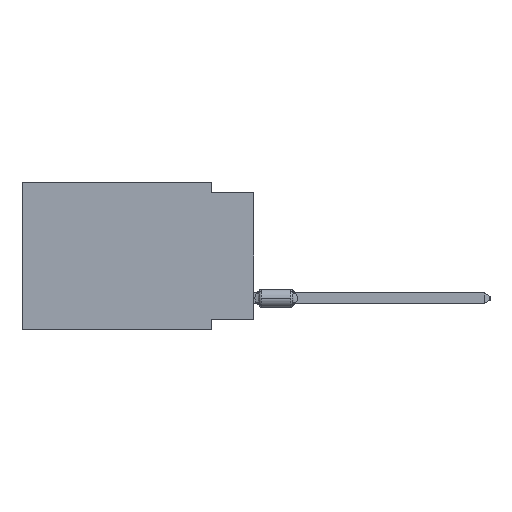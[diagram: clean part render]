
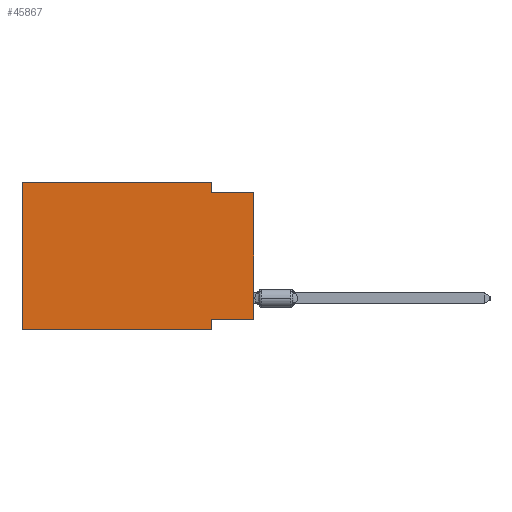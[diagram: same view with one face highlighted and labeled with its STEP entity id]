
A CAD part, left-side view. The second image highlights one B-rep face of the part: STEP entity #45867.
In plain terms, the highlighted planar face has unit normal (-1, 0, 0).
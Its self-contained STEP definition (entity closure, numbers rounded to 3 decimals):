
#582 = EDGE_CURVE ( 'NONE', #38500, #36623, #30276, .T. ) ;
#1065 = LINE ( 'NONE', #19057, #37546 ) ;
#1199 = DIRECTION ( 'NONE',  ( 0., -1., 0. ) ) ;
#1460 = CARTESIAN_POINT ( 'NONE',  ( 0., 0., -8.255 ) ) ;
#1782 = CARTESIAN_POINT ( 'NONE',  ( 0., 2.54, -8.255 ) ) ;
#2269 = ORIENTED_EDGE ( 'NONE', *, *, #8938, .T. ) ;
#3232 = ORIENTED_EDGE ( 'NONE', *, *, #8780, .F. ) ;
#3403 = EDGE_CURVE ( 'NONE', #39735, #17695, #1065, .T. ) ;
#3860 = CARTESIAN_POINT ( 'NONE',  ( 0., 0., 0. ) ) ;
#7436 = CARTESIAN_POINT ( 'NONE',  ( 0., 13.97, -8.89 ) ) ;
#7491 = EDGE_CURVE ( 'NONE', #36623, #39735, #32395, .T. ) ;
#8540 = CARTESIAN_POINT ( 'NONE',  ( 0., 0., -0.635 ) ) ;
#8604 = VECTOR ( 'NONE', #1199, 1000. ) ;
#8780 = EDGE_CURVE ( 'NONE', #17695, #28703, #16199, .T. ) ;
#8938 = EDGE_CURVE ( 'NONE', #14320, #28703, #11062, .T. ) ;
#9602 = ORIENTED_EDGE ( 'NONE', *, *, #34991, .F. ) ;
#10784 = ORIENTED_EDGE ( 'NONE', *, *, #16526, .F. ) ;
#11062 = LINE ( 'NONE', #3860, #13046 ) ;
#11215 = VECTOR ( 'NONE', #39161, 1000. ) ;
#11547 = ORIENTED_EDGE ( 'NONE', *, *, #7491, .F. ) ;
#12225 = CARTESIAN_POINT ( 'NONE',  ( 0., 2.54, -8.89 ) ) ;
#12309 = DIRECTION ( 'NONE',  ( 0., 0., -1. ) ) ;
#12458 = DIRECTION ( 'NONE',  ( 0., 0., -1. ) ) ;
#12946 = CARTESIAN_POINT ( 'NONE',  ( 0., 13.97, 0. ) ) ;
#13046 = VECTOR ( 'NONE', #39642, 1000. ) ;
#14320 = VERTEX_POINT ( 'NONE', #1460 ) ;
#15558 = DIRECTION ( 'NONE',  ( 1., 0., 0. ) ) ;
#15810 = FACE_OUTER_BOUND ( 'NONE', #23708, .T. ) ;
#16199 = LINE ( 'NONE', #34672, #25310 ) ;
#16331 = DIRECTION ( 'NONE',  ( 0., 0., 1. ) ) ;
#16526 = EDGE_CURVE ( 'NONE', #14320, #27132, #22117, .T. ) ;
#17154 = ORIENTED_EDGE ( 'NONE', *, *, #46981, .T. ) ;
#17695 = VERTEX_POINT ( 'NONE', #27170 ) ;
#18897 = VECTOR ( 'NONE', #16331, 1000. ) ;
#19057 = CARTESIAN_POINT ( 'NONE',  ( 0., 2.54, 0. ) ) ;
#20546 = VECTOR ( 'NONE', #33122, 1000. ) ;
#20685 = CARTESIAN_POINT ( 'NONE',  ( 0., 13.97, 0. ) ) ;
#22117 = LINE ( 'NONE', #36731, #20546 ) ;
#22792 = PLANE ( 'NONE',  #24466 ) ;
#23708 = EDGE_LOOP ( 'NONE', ( #2269, #3232, #41286, #11547, #30032, #17154, #9602, #10784 ) ) ;
#24466 = AXIS2_PLACEMENT_3D ( 'NONE', #30471, #15558, #30228 ) ;
#25119 = CARTESIAN_POINT ( 'NONE',  ( 0., 2.54, 0. ) ) ;
#25310 = VECTOR ( 'NONE', #45725, 1000. ) ;
#27132 = VERTEX_POINT ( 'NONE', #1782 ) ;
#27170 = CARTESIAN_POINT ( 'NONE',  ( 0., 2.54, -0.635 ) ) ;
#28703 = VERTEX_POINT ( 'NONE', #8540 ) ;
#30032 = ORIENTED_EDGE ( 'NONE', *, *, #582, .F. ) ;
#30228 = DIRECTION ( 'NONE',  ( 0., 0., -1. ) ) ;
#30276 = LINE ( 'NONE', #12946, #18897 ) ;
#30471 = CARTESIAN_POINT ( 'NONE',  ( 0., 13.97, 0. ) ) ;
#32395 = LINE ( 'NONE', #20685, #11215 ) ;
#33122 = DIRECTION ( 'NONE',  ( 0., 1., 0. ) ) ;
#34672 = CARTESIAN_POINT ( 'NONE',  ( 0., 0., -0.635 ) ) ;
#34991 = EDGE_CURVE ( 'NONE', #27132, #35376, #41295, .T. ) ;
#35376 = VERTEX_POINT ( 'NONE', #41479 ) ;
#36623 = VERTEX_POINT ( 'NONE', #41000 ) ;
#36731 = CARTESIAN_POINT ( 'NONE',  ( 0., 0., -8.255 ) ) ;
#37546 = VECTOR ( 'NONE', #12309, 1000. ) ;
#37798 = VECTOR ( 'NONE', #12458, 1000. ) ;
#38500 = VERTEX_POINT ( 'NONE', #43345 ) ;
#39161 = DIRECTION ( 'NONE',  ( 0., -1., 0. ) ) ;
#39642 = DIRECTION ( 'NONE',  ( 0., 0., 1. ) ) ;
#39735 = VERTEX_POINT ( 'NONE', #25119 ) ;
#40318 = LINE ( 'NONE', #7436, #8604 ) ;
#41000 = CARTESIAN_POINT ( 'NONE',  ( 0., 13.97, 0. ) ) ;
#41286 = ORIENTED_EDGE ( 'NONE', *, *, #3403, .F. ) ;
#41295 = LINE ( 'NONE', #12225, #37798 ) ;
#41479 = CARTESIAN_POINT ( 'NONE',  ( 0., 2.54, -8.89 ) ) ;
#43345 = CARTESIAN_POINT ( 'NONE',  ( 0., 13.97, -8.89 ) ) ;
#45725 = DIRECTION ( 'NONE',  ( 0., -1., 0. ) ) ;
#45867 = ADVANCED_FACE ( 'NONE', ( #15810 ), #22792, .F. ) ;
#46981 = EDGE_CURVE ( 'NONE', #38500, #35376, #40318, .T. ) ;
